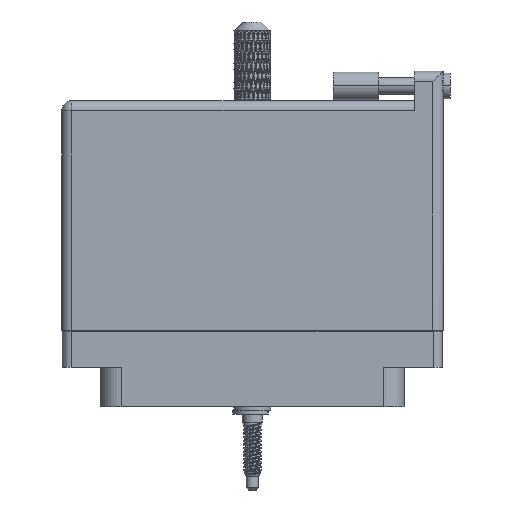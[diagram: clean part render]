
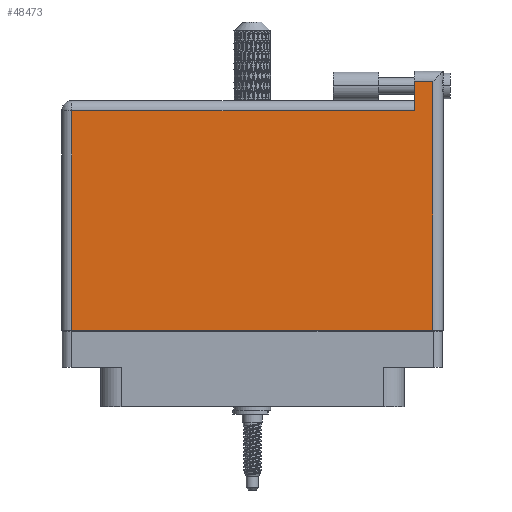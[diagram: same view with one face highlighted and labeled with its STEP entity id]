
A CAD part, front view. The second image highlights one B-rep face of the part: STEP entity #48473.
In plain terms, the highlighted face is planar.
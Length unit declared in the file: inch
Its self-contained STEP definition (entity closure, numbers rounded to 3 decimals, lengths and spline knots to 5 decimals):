
#1236 = ORIENTED_EDGE ( 'NONE', *, *, #57554, .T. ) ;
#2451 = CARTESIAN_POINT ( 'NONE',  ( 1.23, -0.1, 0.4495 ) ) ;
#3790 = PLANE ( 'NONE',  #7533 ) ;
#4532 = FACE_OUTER_BOUND ( 'NONE', #6344, .T. ) ;
#5311 = VECTOR ( 'NONE', #88537, 39.37008 ) ;
#6140 = VECTOR ( 'NONE', #79111, 39.37008 ) ;
#6344 = EDGE_LOOP ( 'NONE', ( #1236, #19467, #117381, #80446, #94129, #70216 ) ) ;
#6950 = EDGE_CURVE ( 'NONE', #56274, #94418, #114024, .T. ) ;
#7533 = AXIS2_PLACEMENT_3D ( 'NONE', #12232, #67242, #22097 ) ;
#11169 = CARTESIAN_POINT ( 'NONE',  ( -1.3, -0.1, 0.4495 ) ) ;
#12232 = CARTESIAN_POINT ( 'NONE',  ( -1.3, 1.466, 0.4495 ) ) ;
#14031 = VERTEX_POINT ( 'NONE', #66520 ) ;
#19467 = ORIENTED_EDGE ( 'NONE', *, *, #21480, .T. ) ;
#20942 = CARTESIAN_POINT ( 'NONE',  ( 1.23, 1.596, 0.4495 ) ) ;
#21480 = EDGE_CURVE ( 'NONE', #67230, #56730, #93225, .T. ) ;
#22097 = DIRECTION ( 'NONE',  ( -1., 0., 0. ) ) ;
#27434 = LINE ( 'NONE', #58214, #6140 ) ;
#29365 = DIRECTION ( 'NONE',  ( 1., 0., 0. ) ) ;
#36265 = LINE ( 'NONE', #70803, #111404 ) ;
#40523 = DIRECTION ( 'NONE',  ( 0., -1., 0. ) ) ;
#41687 = VERTEX_POINT ( 'NONE', #86053 ) ;
#47161 = EDGE_CURVE ( 'NONE', #94418, #14031, #27434, .T. ) ;
#48473 = ADVANCED_FACE ( 'NONE', ( #4532 ), #3790, .F. ) ;
#54446 = LINE ( 'NONE', #68160, #92694 ) ;
#56274 = VERTEX_POINT ( 'NONE', #97138 ) ;
#56730 = VERTEX_POINT ( 'NONE', #20942 ) ;
#57554 = EDGE_CURVE ( 'NONE', #41687, #67230, #64547, .T. ) ;
#58214 = CARTESIAN_POINT ( 'NONE',  ( -1.3, 1.396, 0.4495 ) ) ;
#60229 = DIRECTION ( 'NONE',  ( -1., 0., 0. ) ) ;
#64547 = LINE ( 'NONE', #11169, #104058 ) ;
#66388 = EDGE_CURVE ( 'NONE', #14031, #41687, #36265, .T. ) ;
#66520 = CARTESIAN_POINT ( 'NONE',  ( -1.23, 1.396, 0.4495 ) ) ;
#67230 = VERTEX_POINT ( 'NONE', #2451 ) ;
#67242 = DIRECTION ( 'NONE',  ( 0., 0., -1. ) ) ;
#68160 = CARTESIAN_POINT ( 'NONE',  ( -1.3, 1.596, 0.4495 ) ) ;
#69912 = EDGE_CURVE ( 'NONE', #56730, #56274, #54446, .T. ) ;
#70216 = ORIENTED_EDGE ( 'NONE', *, *, #66388, .T. ) ;
#70803 = CARTESIAN_POINT ( 'NONE',  ( -1.23, -0.1, 0.4495 ) ) ;
#79111 = DIRECTION ( 'NONE',  ( -1., 0., 0. ) ) ;
#79437 = CARTESIAN_POINT ( 'NONE',  ( 1.23, 1.666, 0.4495 ) ) ;
#79512 = DIRECTION ( 'NONE',  ( 0., -1., 0. ) ) ;
#80446 = ORIENTED_EDGE ( 'NONE', *, *, #6950, .T. ) ;
#81470 = VECTOR ( 'NONE', #40523, 39.37008 ) ;
#86053 = CARTESIAN_POINT ( 'NONE',  ( -1.23, -0.1, 0.4495 ) ) ;
#88537 = DIRECTION ( 'NONE',  ( 0., 1., 0. ) ) ;
#92694 = VECTOR ( 'NONE', #60229, 39.37008 ) ;
#93225 = LINE ( 'NONE', #79437, #5311 ) ;
#94129 = ORIENTED_EDGE ( 'NONE', *, *, #47161, .T. ) ;
#94418 = VERTEX_POINT ( 'NONE', #97075 ) ;
#94786 = CARTESIAN_POINT ( 'NONE',  ( 1.103, 1.666, 0.4495 ) ) ;
#97075 = CARTESIAN_POINT ( 'NONE',  ( 1.103, 1.396, 0.4495 ) ) ;
#97138 = CARTESIAN_POINT ( 'NONE',  ( 1.103, 1.596, 0.4495 ) ) ;
#104058 = VECTOR ( 'NONE', #29365, 39.37008 ) ;
#111404 = VECTOR ( 'NONE', #79512, 39.37008 ) ;
#114024 = LINE ( 'NONE', #94786, #81470 ) ;
#117381 = ORIENTED_EDGE ( 'NONE', *, *, #69912, .T. ) ;
